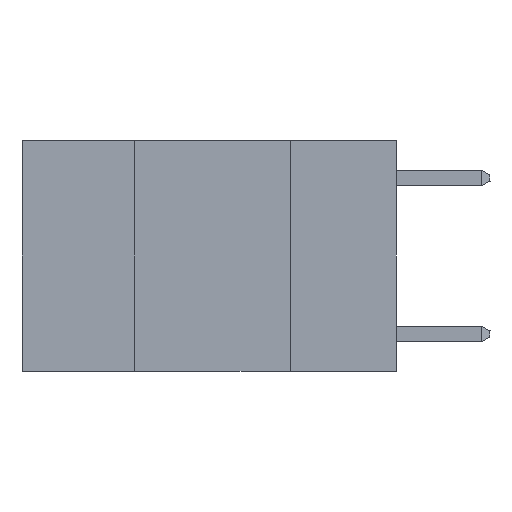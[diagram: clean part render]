
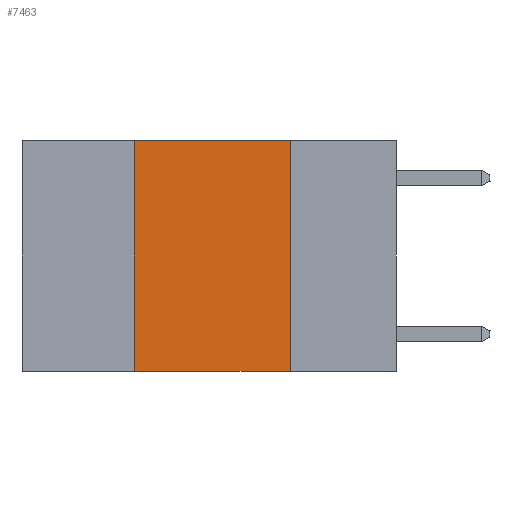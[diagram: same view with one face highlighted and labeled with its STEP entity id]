
A CAD part, left-side view. The second image highlights one B-rep face of the part: STEP entity #7463.
In plain terms, the highlighted planar face has unit normal (-1, 0, 0).
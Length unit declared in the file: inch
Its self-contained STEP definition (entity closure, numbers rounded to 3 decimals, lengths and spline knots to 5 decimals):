
#952 = VECTOR ( 'NONE', #10400, 39.37008 ) ;
#992 = CARTESIAN_POINT ( 'NONE',  ( 0., 0.6, 0. ) ) ;
#1099 = EDGE_CURVE ( 'NONE', #1718, #2143, #2459, .T. ) ;
#1438 = VECTOR ( 'NONE', #9798, 39.37008 ) ;
#1598 = EDGE_CURVE ( 'NONE', #2143, #4845, #3578, .T. ) ;
#1718 = VERTEX_POINT ( 'NONE', #8008 ) ;
#1941 = VECTOR ( 'NONE', #10259, 39.37008 ) ;
#2143 = VERTEX_POINT ( 'NONE', #4703 ) ;
#2253 = LINE ( 'NONE', #9484, #10274 ) ;
#2459 = LINE ( 'NONE', #2491, #1941 ) ;
#2491 = CARTESIAN_POINT ( 'NONE',  ( 0., 0.42, 0. ) ) ;
#2901 = LINE ( 'NONE', #3184, #952 ) ;
#2967 = VERTEX_POINT ( 'NONE', #7587 ) ;
#3184 = CARTESIAN_POINT ( 'NONE',  ( 0., 0.17, 0. ) ) ;
#3248 = FACE_OUTER_BOUND ( 'NONE', #7112, .T. ) ;
#3578 = LINE ( 'NONE', #992, #1438 ) ;
#4011 = DIRECTION ( 'NONE',  ( 0., -1., 0. ) ) ;
#4357 = CARTESIAN_POINT ( 'NONE',  ( 0., 0.17, 0. ) ) ;
#4703 = CARTESIAN_POINT ( 'NONE',  ( 0., 0.42, 0. ) ) ;
#4787 = DIRECTION ( 'NONE',  ( 0., 0., -1. ) ) ;
#4845 = VERTEX_POINT ( 'NONE', #4357 ) ;
#5518 = ORIENTED_EDGE ( 'NONE', *, *, #1598, .F. ) ;
#5542 = AXIS2_PLACEMENT_3D ( 'NONE', #8756, #9528, #4787 ) ;
#5577 = EDGE_CURVE ( 'NONE', #1718, #2967, #2253, .T. ) ;
#6276 = EDGE_CURVE ( 'NONE', #4845, #2967, #2901, .T. ) ;
#7112 = EDGE_LOOP ( 'NONE', ( #8800, #5518, #7605, #9722 ) ) ;
#7463 = ADVANCED_FACE ( 'NONE', ( #3248 ), #7957, .F. ) ;
#7587 = CARTESIAN_POINT ( 'NONE',  ( 0., 0.17, -0.37 ) ) ;
#7605 = ORIENTED_EDGE ( 'NONE', *, *, #1099, .F. ) ;
#7957 = PLANE ( 'NONE',  #5542 ) ;
#8008 = CARTESIAN_POINT ( 'NONE',  ( 0., 0.42, -0.37 ) ) ;
#8756 = CARTESIAN_POINT ( 'NONE',  ( 0., 0.6, 0. ) ) ;
#8800 = ORIENTED_EDGE ( 'NONE', *, *, #6276, .F. ) ;
#9484 = CARTESIAN_POINT ( 'NONE',  ( 0., 0.6, -0.37 ) ) ;
#9528 = DIRECTION ( 'NONE',  ( 1., 0., 0. ) ) ;
#9722 = ORIENTED_EDGE ( 'NONE', *, *, #5577, .T. ) ;
#9798 = DIRECTION ( 'NONE',  ( 0., -1., 0. ) ) ;
#10259 = DIRECTION ( 'NONE',  ( 0., 0., 1. ) ) ;
#10274 = VECTOR ( 'NONE', #4011, 39.37008 ) ;
#10400 = DIRECTION ( 'NONE',  ( 0., 0., -1. ) ) ;
